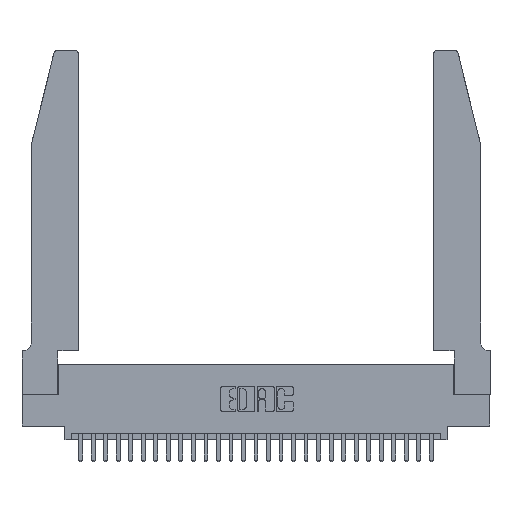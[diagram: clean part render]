
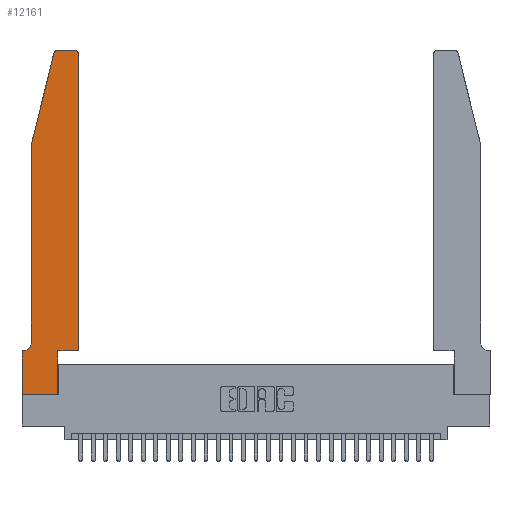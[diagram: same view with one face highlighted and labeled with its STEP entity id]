
A CAD part, top view. The second image highlights one B-rep face of the part: STEP entity #12161.
In plain terms, the highlighted planar face has unit normal (0, 0, 1).
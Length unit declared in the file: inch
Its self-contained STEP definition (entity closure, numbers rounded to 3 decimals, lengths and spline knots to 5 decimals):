
#117 = DIRECTION ( 'NONE',  ( -1., 0., 0. ) ) ;
#190 = DIRECTION ( 'NONE',  ( 0., -1., 0. ) ) ;
#256 = VERTEX_POINT ( 'NONE', #7713 ) ;
#599 = VERTEX_POINT ( 'NONE', #26545 ) ;
#1238 = DIRECTION ( 'NONE',  ( 1., 0., 0. ) ) ;
#1352 = AXIS2_PLACEMENT_3D ( 'NONE', #19631, #5868, #21988 ) ;
#2162 = VERTEX_POINT ( 'NONE', #16060 ) ;
#2895 = CARTESIAN_POINT ( 'NONE',  ( 0., 0., 0.37 ) ) ;
#3320 = DIRECTION ( 'NONE',  ( 1., 0., 0. ) ) ;
#3717 = DIRECTION ( 'NONE',  ( 0., 0., 1. ) ) ;
#4842 = PLANE ( 'NONE',  #23378 ) ;
#5200 = CARTESIAN_POINT ( 'NONE',  ( 0.2865, 0.35, 0.37 ) ) ;
#5548 = LINE ( 'NONE', #5200, #29077 ) ;
#5699 = EDGE_CURVE ( 'NONE', #18442, #22891, #26922, .T. ) ;
#5822 = CARTESIAN_POINT ( 'NONE',  ( 0., 0.35, 0.37 ) ) ;
#5868 = DIRECTION ( 'NONE',  ( 0., 0., 1. ) ) ;
#5918 = DIRECTION ( 'NONE',  ( 1., 0., 0. ) ) ;
#5975 = VERTEX_POINT ( 'NONE', #12747 ) ;
#6002 = VECTOR ( 'NONE', #190, 39.37008 ) ;
#6112 = CARTESIAN_POINT ( 'NONE',  ( 0., 0., 0.37 ) ) ;
#6400 = ORIENTED_EDGE ( 'NONE', *, *, #6827, .T. ) ;
#6827 = EDGE_CURVE ( 'NONE', #7327, #5975, #10089, .T. ) ;
#7189 = DIRECTION ( 'NONE',  ( 0., -1., 0. ) ) ;
#7327 = VERTEX_POINT ( 'NONE', #6112 ) ;
#7540 = LINE ( 'NONE', #2895, #7929 ) ;
#7586 = CARTESIAN_POINT ( 'NONE',  ( 0.4505, 0.35, 0.37 ) ) ;
#7649 = VECTOR ( 'NONE', #10344, 39.37008 ) ;
#7713 = CARTESIAN_POINT ( 'NONE',  ( 0.2865, 0.35, 0.37 ) ) ;
#7902 = ORIENTED_EDGE ( 'NONE', *, *, #25822, .T. ) ;
#7929 = VECTOR ( 'NONE', #7189, 39.37008 ) ;
#8353 = VECTOR ( 'NONE', #1238, 39.37008 ) ;
#8697 = LINE ( 'NONE', #7586, #22981 ) ;
#9213 = CARTESIAN_POINT ( 'NONE',  ( 0.0755, 2., 0.37 ) ) ;
#9252 = VECTOR ( 'NONE', #28469, 39.37008 ) ;
#10059 = DIRECTION ( 'NONE',  ( 1., 0., 0. ) ) ;
#10086 = EDGE_CURVE ( 'NONE', #13259, #24870, #14587, .T. ) ;
#10089 = LINE ( 'NONE', #24524, #8353 ) ;
#10184 = DIRECTION ( 'NONE',  ( 0., 0., 1. ) ) ;
#10344 = DIRECTION ( 'NONE',  ( -0.239, -0.971, 0. ) ) ;
#10923 = CIRCLE ( 'NONE', #18608, 0.07 ) ;
#11535 = EDGE_CURVE ( 'NONE', #22891, #26379, #13110, .T. ) ;
#12007 = ORIENTED_EDGE ( 'NONE', *, *, #17932, .T. ) ;
#12161 = ADVANCED_FACE ( 'NONE', ( #15230 ), #4842, .T. ) ;
#12344 = CARTESIAN_POINT ( 'NONE',  ( 0.4505, 2.72, 0.37 ) ) ;
#12354 = CARTESIAN_POINT ( 'NONE',  ( 0.284, 2.75, 0.37 ) ) ;
#12747 = CARTESIAN_POINT ( 'NONE',  ( 0.2865, 0., 0.37 ) ) ;
#12973 = ORIENTED_EDGE ( 'NONE', *, *, #26820, .T. ) ;
#13110 = CIRCLE ( 'NONE', #25091, 0.03 ) ;
#13259 = VERTEX_POINT ( 'NONE', #12354 ) ;
#14018 = ORIENTED_EDGE ( 'NONE', *, *, #25993, .T. ) ;
#14587 = CIRCLE ( 'NONE', #1352, 0.03 ) ;
#14851 = LINE ( 'NONE', #15897, #25498 ) ;
#15058 = CARTESIAN_POINT ( 'NONE',  ( 0.2605, 2.75, 0.37 ) ) ;
#15185 = VECTOR ( 'NONE', #18624, 39.37008 ) ;
#15229 = CARTESIAN_POINT ( 'NONE',  ( 0.4205, 2.72, 0.37 ) ) ;
#15230 = FACE_OUTER_BOUND ( 'NONE', #23875, .T. ) ;
#15385 = LINE ( 'NONE', #15058, #9252 ) ;
#15775 = CARTESIAN_POINT ( 'NONE',  ( 0.4205, 2.75, 0.37 ) ) ;
#15897 = CARTESIAN_POINT ( 'NONE',  ( 0.0755, 0.35, 0.37 ) ) ;
#16055 = VERTEX_POINT ( 'NONE', #23639 ) ;
#16060 = CARTESIAN_POINT ( 'NONE',  ( 0.0055, 0.35, 0.37 ) ) ;
#16089 = EDGE_CURVE ( 'NONE', #256, #18442, #8697, .T. ) ;
#16329 = CARTESIAN_POINT ( 'NONE',  ( 0.4505, 0.35, 0.37 ) ) ;
#16506 = ORIENTED_EDGE ( 'NONE', *, *, #5699, .T. ) ;
#16619 = ORIENTED_EDGE ( 'NONE', *, *, #22561, .T. ) ;
#16930 = CARTESIAN_POINT ( 'NONE',  ( 0.25487, 2.72718, 0.37 ) ) ;
#17160 = VERTEX_POINT ( 'NONE', #9213 ) ;
#17932 = EDGE_CURVE ( 'NONE', #599, #7327, #7540, .T. ) ;
#18442 = VERTEX_POINT ( 'NONE', #25211 ) ;
#18608 = AXIS2_PLACEMENT_3D ( 'NONE', #24186, #21813, #28558 ) ;
#18624 = DIRECTION ( 'NONE',  ( 0., 1., 0. ) ) ;
#18678 = DIRECTION ( 'NONE',  ( 0., 1., 0. ) ) ;
#19147 = ORIENTED_EDGE ( 'NONE', *, *, #11535, .T. ) ;
#19631 = CARTESIAN_POINT ( 'NONE',  ( 0.284, 2.72, 0.37 ) ) ;
#19643 = ORIENTED_EDGE ( 'NONE', *, *, #10086, .T. ) ;
#20854 = LINE ( 'NONE', #24019, #7649 ) ;
#20994 = LINE ( 'NONE', #25210, #6002 ) ;
#21813 = DIRECTION ( 'NONE',  ( 0., 0., -1. ) ) ;
#21988 = DIRECTION ( 'NONE',  ( 1., 0., 0. ) ) ;
#22561 = EDGE_CURVE ( 'NONE', #26379, #13259, #15385, .T. ) ;
#22891 = VERTEX_POINT ( 'NONE', #12344 ) ;
#22981 = VECTOR ( 'NONE', #10059, 39.37008 ) ;
#23378 = AXIS2_PLACEMENT_3D ( 'NONE', #5822, #3717, #5918 ) ;
#23639 = CARTESIAN_POINT ( 'NONE',  ( 0.0755, 0.42, 0.37 ) ) ;
#23875 = EDGE_LOOP ( 'NONE', ( #16619, #19643, #24869, #24639, #12973, #7902, #12007, #6400, #14018, #26782, #16506, #19147 ) ) ;
#24019 = CARTESIAN_POINT ( 'NONE',  ( 0.0755, 2., 0.37 ) ) ;
#24107 = EDGE_CURVE ( 'NONE', #17160, #16055, #20994, .T. ) ;
#24186 = CARTESIAN_POINT ( 'NONE',  ( 0.0055, 0.42, 0.37 ) ) ;
#24524 = CARTESIAN_POINT ( 'NONE',  ( 0., 0., 0.37 ) ) ;
#24639 = ORIENTED_EDGE ( 'NONE', *, *, #24107, .T. ) ;
#24869 = ORIENTED_EDGE ( 'NONE', *, *, #26178, .T. ) ;
#24870 = VERTEX_POINT ( 'NONE', #16930 ) ;
#25091 = AXIS2_PLACEMENT_3D ( 'NONE', #15229, #10184, #3320 ) ;
#25210 = CARTESIAN_POINT ( 'NONE',  ( 0.0755, 2., 0.37 ) ) ;
#25211 = CARTESIAN_POINT ( 'NONE',  ( 0.4505, 0.35, 0.37 ) ) ;
#25498 = VECTOR ( 'NONE', #117, 39.37008 ) ;
#25822 = EDGE_CURVE ( 'NONE', #2162, #599, #14851, .T. ) ;
#25993 = EDGE_CURVE ( 'NONE', #5975, #256, #5548, .T. ) ;
#26178 = EDGE_CURVE ( 'NONE', #24870, #17160, #20854, .T. ) ;
#26379 = VERTEX_POINT ( 'NONE', #15775 ) ;
#26545 = CARTESIAN_POINT ( 'NONE',  ( 0., 0.35, 0.37 ) ) ;
#26782 = ORIENTED_EDGE ( 'NONE', *, *, #16089, .T. ) ;
#26820 = EDGE_CURVE ( 'NONE', #16055, #2162, #10923, .T. ) ;
#26922 = LINE ( 'NONE', #16329, #15185 ) ;
#28469 = DIRECTION ( 'NONE',  ( -1., 0., 0. ) ) ;
#28558 = DIRECTION ( 'NONE',  ( -1., 0., 0. ) ) ;
#29077 = VECTOR ( 'NONE', #18678, 39.37008 ) ;
